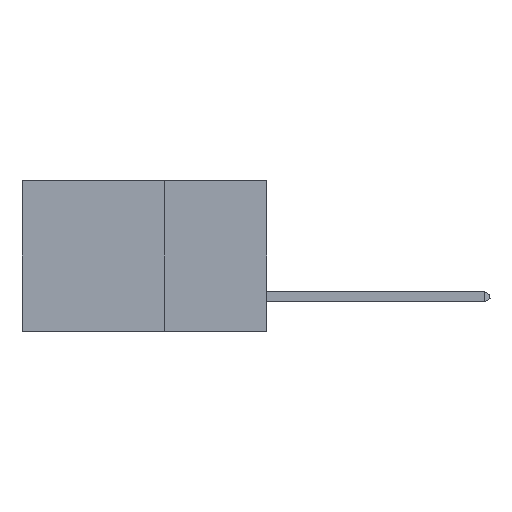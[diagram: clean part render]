
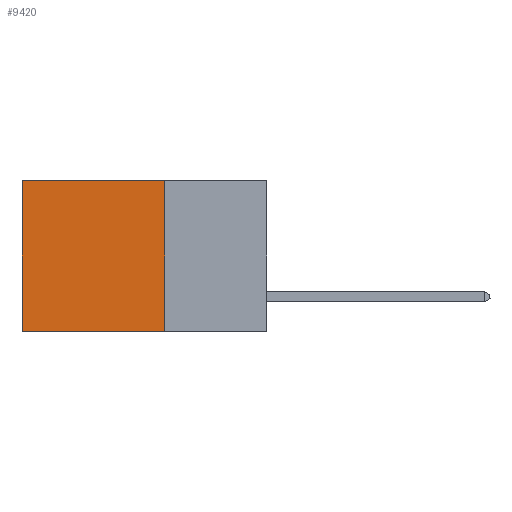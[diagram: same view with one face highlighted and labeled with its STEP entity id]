
A CAD part, left-side view. The second image highlights one B-rep face of the part: STEP entity #9420.
In plain terms, the highlighted planar face has unit normal (-1, 0, 0).
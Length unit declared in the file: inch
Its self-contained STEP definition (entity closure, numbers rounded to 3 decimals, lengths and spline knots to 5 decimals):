
#877 = LINE ( 'NONE', #10615, #16949 ) ;
#1791 = DIRECTION ( 'NONE',  ( 0., 1., 0. ) ) ;
#2266 = VERTEX_POINT ( 'NONE', #11217 ) ;
#3503 = DIRECTION ( 'NONE',  ( 0., 1., 0. ) ) ;
#3784 = CARTESIAN_POINT ( 'NONE',  ( 0.2875, 0.25, 0. ) ) ;
#4537 = CARTESIAN_POINT ( 'NONE',  ( 0.2875, 0.6, 0. ) ) ;
#4937 = EDGE_CURVE ( 'NONE', #18762, #10705, #5591, .T. ) ;
#5322 = VECTOR ( 'NONE', #14587, 39.37008 ) ;
#5373 = AXIS2_PLACEMENT_3D ( 'NONE', #3784, #18592, #15728 ) ;
#5591 = LINE ( 'NONE', #6508, #7934 ) ;
#5890 = CARTESIAN_POINT ( 'NONE',  ( 0.2875, 0.25, -0.37 ) ) ;
#6508 = CARTESIAN_POINT ( 'NONE',  ( 0.2875, 0.25, -0.37 ) ) ;
#6952 = LINE ( 'NONE', #7456, #15341 ) ;
#7221 = EDGE_CURVE ( 'NONE', #19234, #10705, #16762, .T. ) ;
#7456 = CARTESIAN_POINT ( 'NONE',  ( 0.2875, 0.25, 0. ) ) ;
#7934 = VECTOR ( 'NONE', #3503, 39.37008 ) ;
#8912 = EDGE_CURVE ( 'NONE', #2266, #18762, #877, .T. ) ;
#9420 = ADVANCED_FACE ( 'NONE', ( #12502 ), #9788, .F. ) ;
#9788 = PLANE ( 'NONE',  #5373 ) ;
#10142 = CARTESIAN_POINT ( 'NONE',  ( 0.2875, 0.6, -0.37 ) ) ;
#10615 = CARTESIAN_POINT ( 'NONE',  ( 0.2875, 0.25, 0. ) ) ;
#10705 = VERTEX_POINT ( 'NONE', #10142 ) ;
#11217 = CARTESIAN_POINT ( 'NONE',  ( 0.2875, 0.25, 0. ) ) ;
#12414 = ORIENTED_EDGE ( 'NONE', *, *, #4937, .F. ) ;
#12463 = EDGE_LOOP ( 'NONE', ( #14588, #12414, #17643, #18874 ) ) ;
#12502 = FACE_OUTER_BOUND ( 'NONE', #12463, .T. ) ;
#13414 = DIRECTION ( 'NONE',  ( 0., 0., -1. ) ) ;
#14587 = DIRECTION ( 'NONE',  ( 0., 0., -1. ) ) ;
#14588 = ORIENTED_EDGE ( 'NONE', *, *, #7221, .T. ) ;
#15341 = VECTOR ( 'NONE', #1791, 39.37008 ) ;
#15728 = DIRECTION ( 'NONE',  ( 0., 0., -1. ) ) ;
#16762 = LINE ( 'NONE', #17513, #5322 ) ;
#16949 = VECTOR ( 'NONE', #13414, 39.37008 ) ;
#17513 = CARTESIAN_POINT ( 'NONE',  ( 0.2875, 0.6, 0. ) ) ;
#17643 = ORIENTED_EDGE ( 'NONE', *, *, #8912, .F. ) ;
#18592 = DIRECTION ( 'NONE',  ( 1., 0., 0. ) ) ;
#18762 = VERTEX_POINT ( 'NONE', #5890 ) ;
#18776 = EDGE_CURVE ( 'NONE', #2266, #19234, #6952, .T. ) ;
#18874 = ORIENTED_EDGE ( 'NONE', *, *, #18776, .T. ) ;
#19234 = VERTEX_POINT ( 'NONE', #4537 ) ;
